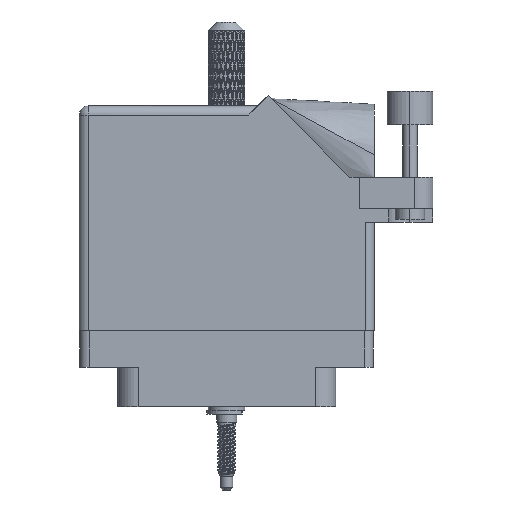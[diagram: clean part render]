
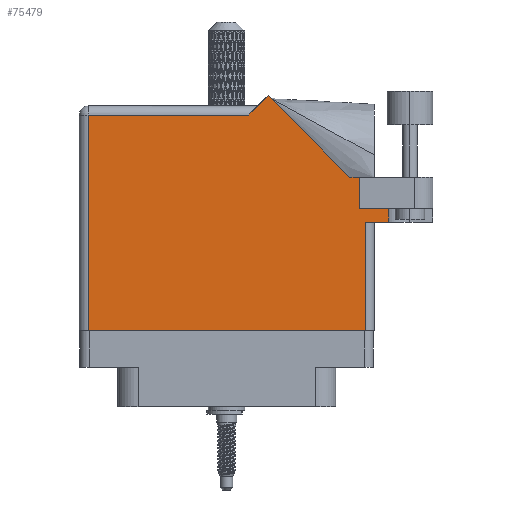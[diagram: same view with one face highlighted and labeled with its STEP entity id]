
A CAD part, front view. The second image highlights one B-rep face of the part: STEP entity #75479.
In plain terms, the highlighted face is planar.
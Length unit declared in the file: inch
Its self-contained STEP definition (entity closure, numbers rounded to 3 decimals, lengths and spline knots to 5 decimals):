
#2155 = VECTOR ( 'NONE', #90598, 39.37008 ) ;
#2708 = ORIENTED_EDGE ( 'NONE', *, *, #6745, .T. ) ;
#3524 = LINE ( 'NONE', #26033, #2155 ) ;
#3561 = VECTOR ( 'NONE', #23016, 39.37008 ) ;
#3667 = LINE ( 'NONE', #12219, #14000 ) ;
#5044 = CARTESIAN_POINT ( 'NONE',  ( 0.943, -0.1, 0.455 ) ) ;
#6745 = EDGE_CURVE ( 'NONE', #57939, #34509, #56203, .T. ) ;
#6799 = ORIENTED_EDGE ( 'NONE', *, *, #31971, .T. ) ;
#7309 = EDGE_CURVE ( 'NONE', #21383, #19771, #84436, .T. ) ;
#7756 = DIRECTION ( 'NONE',  ( -1., 0., 0. ) ) ;
#8493 = CARTESIAN_POINT ( 'NONE',  ( -0.943, 1.368, 0.455 ) ) ;
#9070 = EDGE_CURVE ( 'NONE', #88221, #87447, #83061, .T. ) ;
#11625 = CARTESIAN_POINT ( 'NONE',  ( 0.212, 1.43, 0.455 ) ) ;
#11928 = CARTESIAN_POINT ( 'NONE',  ( 0.83942, 0.944, 0.455 ) ) ;
#11945 = EDGE_CURVE ( 'NONE', #98719, #88221, #101091, .T. ) ;
#12219 = CARTESIAN_POINT ( 'NONE',  ( -0.943, -0.1, 0.455 ) ) ;
#12341 = LINE ( 'NONE', #13926, #23823 ) ;
#13926 = CARTESIAN_POINT ( 'NONE',  ( 1.405, 0.944, 0.455 ) ) ;
#14000 = VECTOR ( 'NONE', #85056, 39.37008 ) ;
#15062 = ORIENTED_EDGE ( 'NONE', *, *, #55763, .T. ) ;
#15326 = CARTESIAN_POINT ( 'NONE',  ( 0.83942, 0.944, 0.455 ) ) ;
#17280 = CARTESIAN_POINT ( 'NONE',  ( 0.943, 0.637, 0.455 ) ) ;
#19771 = VERTEX_POINT ( 'NONE', #55655 ) ;
#19785 = ORIENTED_EDGE ( 'NONE', *, *, #11945, .T. ) ;
#21328 = LINE ( 'NONE', #97113, #48264 ) ;
#21383 = VERTEX_POINT ( 'NONE', #5044 ) ;
#23016 = DIRECTION ( 'NONE',  ( -0.707, 0.707, 0. ) ) ;
#23823 = VECTOR ( 'NONE', #28964, 39.37008 ) ;
#26033 = CARTESIAN_POINT ( 'NONE',  ( 1.1065, 1.06177, 0.455 ) ) ;
#28009 = DIRECTION ( 'NONE',  ( -1., 0., 0. ) ) ;
#28444 = CARTESIAN_POINT ( 'NONE',  ( -0.943, -0.1, 0.455 ) ) ;
#28964 = DIRECTION ( 'NONE',  ( -1., 0., 0. ) ) ;
#29174 = VECTOR ( 'NONE', #94904, 39.37008 ) ;
#29238 = ORIENTED_EDGE ( 'NONE', *, *, #75110, .T. ) ;
#30195 = CARTESIAN_POINT ( 'NONE',  ( 0.905, 0.731, 0.455 ) ) ;
#31552 = CARTESIAN_POINT ( 'NONE',  ( 1.005, 0.637, 0.455 ) ) ;
#31971 = EDGE_CURVE ( 'NONE', #55371, #21383, #45909, .T. ) ;
#33707 = DIRECTION ( 'NONE',  ( 0., 1., 0. ) ) ;
#34509 = VERTEX_POINT ( 'NONE', #103871 ) ;
#35210 = PLANE ( 'NONE',  #72830 ) ;
#35907 = CARTESIAN_POINT ( 'NONE',  ( -1.005, 1.43, 0.455 ) ) ;
#40953 = ORIENTED_EDGE ( 'NONE', *, *, #65810, .T. ) ;
#41517 = EDGE_CURVE ( 'NONE', #57939, #62113, #53662, .T. ) ;
#45909 = LINE ( 'NONE', #79339, #89579 ) ;
#46958 = FACE_OUTER_BOUND ( 'NONE', #57005, .T. ) ;
#47204 = VECTOR ( 'NONE', #48453, 39.37008 ) ;
#48264 = VECTOR ( 'NONE', #7756, 39.37008 ) ;
#48453 = DIRECTION ( 'NONE',  ( 0., 1., 0. ) ) ;
#50991 = ORIENTED_EDGE ( 'NONE', *, *, #68027, .T. ) ;
#53662 = LINE ( 'NONE', #87391, #29174 ) ;
#55371 = VERTEX_POINT ( 'NONE', #28444 ) ;
#55655 = CARTESIAN_POINT ( 'NONE',  ( 0.943, 0.637, 0.455 ) ) ;
#55763 = EDGE_CURVE ( 'NONE', #66212, #55371, #3667, .T. ) ;
#56203 = LINE ( 'NONE', #96940, #47204 ) ;
#57005 = EDGE_LOOP ( 'NONE', ( #6799, #97660, #40953, #74286, #89778, #2708, #29238, #19785, #75808, #50991, #15062 ) ) ;
#57939 = VERTEX_POINT ( 'NONE', #30195 ) ;
#58312 = CARTESIAN_POINT ( 'NONE',  ( 1.1065, 0.731, 0.455 ) ) ;
#61108 = CARTESIAN_POINT ( 'NONE',  ( 0.28271, 1.50071, 0.455 ) ) ;
#62113 = VERTEX_POINT ( 'NONE', #58312 ) ;
#65300 = DIRECTION ( 'NONE',  ( 1., 0., 0. ) ) ;
#65810 = EDGE_CURVE ( 'NONE', #19771, #83575, #101155, .T. ) ;
#66212 = VERTEX_POINT ( 'NONE', #8493 ) ;
#66914 = EDGE_CURVE ( 'NONE', #62113, #83575, #3524, .T. ) ;
#68027 = EDGE_CURVE ( 'NONE', #87447, #66212, #21328, .T. ) ;
#68871 = VECTOR ( 'NONE', #101604, 39.37008 ) ;
#70426 = VECTOR ( 'NONE', #65300, 39.37008 ) ;
#72830 = AXIS2_PLACEMENT_3D ( 'NONE', #35907, #92583, #28009 ) ;
#74286 = ORIENTED_EDGE ( 'NONE', *, *, #66914, .F. ) ;
#75110 = EDGE_CURVE ( 'NONE', #34509, #98719, #12341, .T. ) ;
#75479 = ADVANCED_FACE ( 'NONE', ( #46958 ), #35210, .F. ) ;
#75808 = ORIENTED_EDGE ( 'NONE', *, *, #9070, .T. ) ;
#77400 = CARTESIAN_POINT ( 'NONE',  ( 1.1065, 0.637, 0.455 ) ) ;
#79339 = CARTESIAN_POINT ( 'NONE',  ( -1.005, -0.1, 0.455 ) ) ;
#83061 = LINE ( 'NONE', #11625, #68871 ) ;
#83575 = VERTEX_POINT ( 'NONE', #77400 ) ;
#84436 = LINE ( 'NONE', #17280, #92097 ) ;
#85056 = DIRECTION ( 'NONE',  ( 0., -1., 0. ) ) ;
#87391 = CARTESIAN_POINT ( 'NONE',  ( 0.905, 0.731, 0.455 ) ) ;
#87447 = VERTEX_POINT ( 'NONE', #93994 ) ;
#88221 = VERTEX_POINT ( 'NONE', #61108 ) ;
#89579 = VECTOR ( 'NONE', #95811, 39.37008 ) ;
#89778 = ORIENTED_EDGE ( 'NONE', *, *, #41517, .F. ) ;
#90598 = DIRECTION ( 'NONE',  ( 0., -1., 0. ) ) ;
#92097 = VECTOR ( 'NONE', #33707, 39.37008 ) ;
#92583 = DIRECTION ( 'NONE',  ( 0., 0., -1. ) ) ;
#93994 = CARTESIAN_POINT ( 'NONE',  ( 0.15, 1.368, 0.455 ) ) ;
#94904 = DIRECTION ( 'NONE',  ( 1., 0., 0. ) ) ;
#95811 = DIRECTION ( 'NONE',  ( 1., 0., 0. ) ) ;
#96940 = CARTESIAN_POINT ( 'NONE',  ( 0.905, 0.731, 0.455 ) ) ;
#97113 = CARTESIAN_POINT ( 'NONE',  ( -1.005, 1.368, 0.455 ) ) ;
#97660 = ORIENTED_EDGE ( 'NONE', *, *, #7309, .T. ) ;
#98719 = VERTEX_POINT ( 'NONE', #15326 ) ;
#101091 = LINE ( 'NONE', #11928, #3561 ) ;
#101155 = LINE ( 'NONE', #31552, #70426 ) ;
#101604 = DIRECTION ( 'NONE',  ( -0.707, -0.707, 0. ) ) ;
#103871 = CARTESIAN_POINT ( 'NONE',  ( 0.905, 0.944, 0.455 ) ) ;
